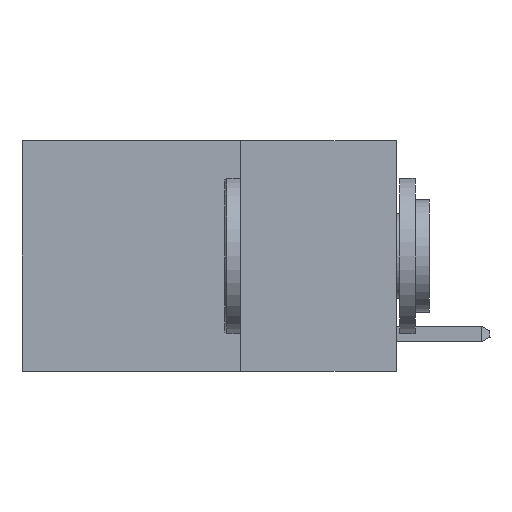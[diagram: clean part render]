
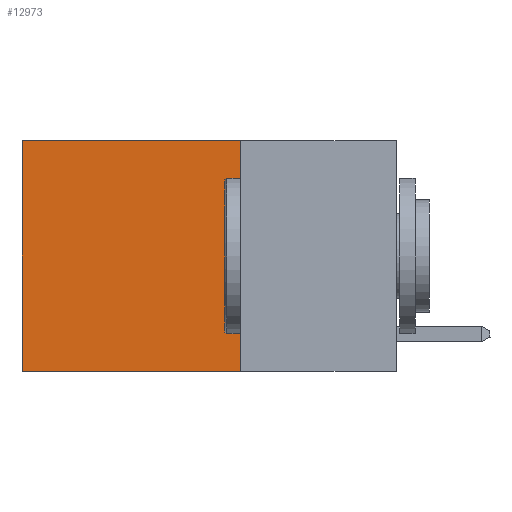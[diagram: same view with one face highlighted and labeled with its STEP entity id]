
A CAD part, left-side view. The second image highlights one B-rep face of the part: STEP entity #12973.
In plain terms, the highlighted planar face has unit normal (-1, 0, 0).
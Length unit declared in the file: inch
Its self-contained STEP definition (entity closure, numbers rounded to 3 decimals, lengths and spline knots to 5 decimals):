
#125 = AXIS2_PLACEMENT_3D ( 'NONE', #18071, #9522, #1006 ) ;
#862 = EDGE_CURVE ( 'NONE', #11013, #15633, #10103, .T. ) ;
#938 = PLANE ( 'NONE',  #125 ) ;
#1006 = DIRECTION ( 'NONE',  ( 0., 0., -1. ) ) ;
#3057 = ORIENTED_EDGE ( 'NONE', *, *, #3547, .T. ) ;
#3132 = LINE ( 'NONE', #13690, #9598 ) ;
#3463 = DIRECTION ( 'NONE',  ( 0., 1., 0. ) ) ;
#3547 = EDGE_CURVE ( 'NONE', #15633, #13636, #16939, .T. ) ;
#3759 = DIRECTION ( 'NONE',  ( 0., 0., -1. ) ) ;
#4677 = CARTESIAN_POINT ( 'NONE',  ( 0.2625, 0.25, -0.37 ) ) ;
#5864 = CARTESIAN_POINT ( 'NONE',  ( 0.2625, 0.25, 0. ) ) ;
#5881 = VECTOR ( 'NONE', #16996, 39.37008 ) ;
#5882 = LINE ( 'NONE', #11996, #13440 ) ;
#5954 = DIRECTION ( 'NONE',  ( 0., 0., -1. ) ) ;
#6026 = VECTOR ( 'NONE', #5954, 39.37008 ) ;
#7867 = VERTEX_POINT ( 'NONE', #4677 ) ;
#8480 = CARTESIAN_POINT ( 'NONE',  ( 0.2625, 0.25, 0. ) ) ;
#9522 = DIRECTION ( 'NONE',  ( 1., 0., 0. ) ) ;
#9598 = VECTOR ( 'NONE', #3759, 39.37008 ) ;
#10103 = LINE ( 'NONE', #8480, #5881 ) ;
#10248 = CARTESIAN_POINT ( 'NONE',  ( 0.2625, 0.6, 0. ) ) ;
#11013 = VERTEX_POINT ( 'NONE', #5864 ) ;
#11996 = CARTESIAN_POINT ( 'NONE',  ( 0.2625, 0.25, -0.37 ) ) ;
#12080 = CARTESIAN_POINT ( 'NONE',  ( 0.2625, 0.6, 0. ) ) ;
#12915 = ORIENTED_EDGE ( 'NONE', *, *, #16991, .F. ) ;
#12973 = ADVANCED_FACE ( 'NONE', ( #17149 ), #938, .F. ) ;
#13440 = VECTOR ( 'NONE', #3463, 39.37008 ) ;
#13636 = VERTEX_POINT ( 'NONE', #13888 ) ;
#13690 = CARTESIAN_POINT ( 'NONE',  ( 0.2625, 0.25, 0. ) ) ;
#13888 = CARTESIAN_POINT ( 'NONE',  ( 0.2625, 0.6, -0.37 ) ) ;
#14299 = ORIENTED_EDGE ( 'NONE', *, *, #17684, .F. ) ;
#15075 = EDGE_LOOP ( 'NONE', ( #3057, #12915, #14299, #16410 ) ) ;
#15633 = VERTEX_POINT ( 'NONE', #12080 ) ;
#16410 = ORIENTED_EDGE ( 'NONE', *, *, #862, .T. ) ;
#16939 = LINE ( 'NONE', #10248, #6026 ) ;
#16991 = EDGE_CURVE ( 'NONE', #7867, #13636, #5882, .T. ) ;
#16996 = DIRECTION ( 'NONE',  ( 0., 1., 0. ) ) ;
#17149 = FACE_OUTER_BOUND ( 'NONE', #15075, .T. ) ;
#17684 = EDGE_CURVE ( 'NONE', #11013, #7867, #3132, .T. ) ;
#18071 = CARTESIAN_POINT ( 'NONE',  ( 0.2625, 0.25, 0. ) ) ;
